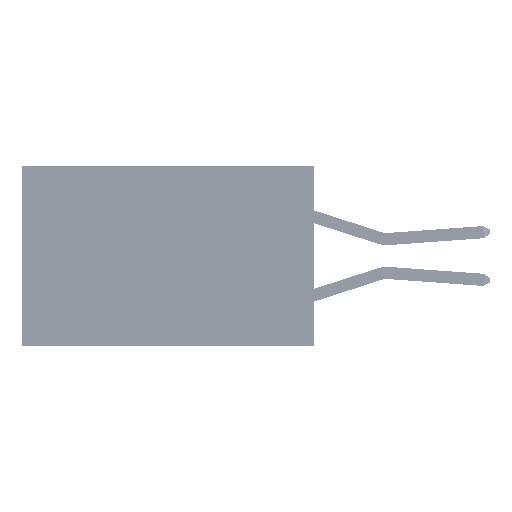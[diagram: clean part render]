
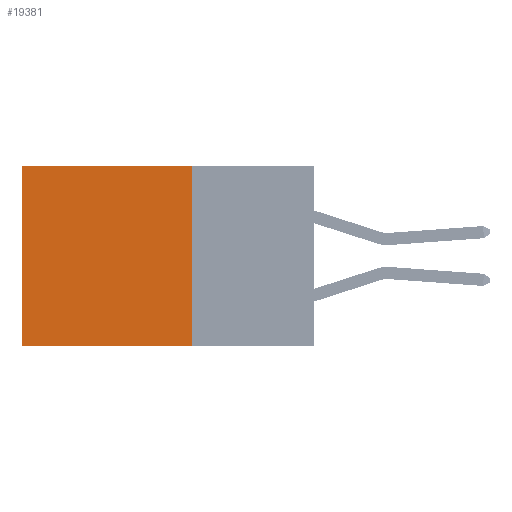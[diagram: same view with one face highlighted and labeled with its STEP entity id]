
A CAD part, left-side view. The second image highlights one B-rep face of the part: STEP entity #19381.
In plain terms, the highlighted planar face has unit normal (-1, 0, 0).
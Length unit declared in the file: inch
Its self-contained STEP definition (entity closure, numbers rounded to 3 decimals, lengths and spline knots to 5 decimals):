
#214 = VERTEX_POINT ( 'NONE', #16503 ) ;
#2511 = ORIENTED_EDGE ( 'NONE', *, *, #20797, .T. ) ;
#3093 = PLANE ( 'NONE',  #17637 ) ;
#3912 = DIRECTION ( 'NONE',  ( 0., 0., -1. ) ) ;
#6927 = DIRECTION ( 'NONE',  ( 1., 0., 0. ) ) ;
#7312 = DIRECTION ( 'NONE',  ( 0., 1., 0. ) ) ;
#7594 = LINE ( 'NONE', #33003, #8791 ) ;
#8791 = VECTOR ( 'NONE', #10518, 39.37008 ) ;
#9837 = LINE ( 'NONE', #20962, #28636 ) ;
#10518 = DIRECTION ( 'NONE',  ( 0., 0., -1. ) ) ;
#10576 = CARTESIAN_POINT ( 'NONE',  ( 0.2875, 0.25, 0. ) ) ;
#12456 = VERTEX_POINT ( 'NONE', #47405 ) ;
#16503 = CARTESIAN_POINT ( 'NONE',  ( 0.2875, 0.6, 0. ) ) ;
#17637 = AXIS2_PLACEMENT_3D ( 'NONE', #10576, #6927, #33221 ) ;
#19381 = ADVANCED_FACE ( 'NONE', ( #26759 ), #3093, .F. ) ;
#19738 = VERTEX_POINT ( 'NONE', #38756 ) ;
#20797 = EDGE_CURVE ( 'NONE', #19738, #214, #40664, .T. ) ;
#20962 = CARTESIAN_POINT ( 'NONE',  ( 0.2875, 0.25, -0.37 ) ) ;
#21660 = VERTEX_POINT ( 'NONE', #47685 ) ;
#22228 = ORIENTED_EDGE ( 'NONE', *, *, #28648, .F. ) ;
#26374 = VECTOR ( 'NONE', #3912, 39.37008 ) ;
#26486 = CARTESIAN_POINT ( 'NONE',  ( 0.2875, 0.6, 0. ) ) ;
#26759 = FACE_OUTER_BOUND ( 'NONE', #41719, .T. ) ;
#28636 = VECTOR ( 'NONE', #35816, 39.37008 ) ;
#28648 = EDGE_CURVE ( 'NONE', #12456, #21660, #9837, .T. ) ;
#30365 = ORIENTED_EDGE ( 'NONE', *, *, #33976, .T. ) ;
#30696 = VECTOR ( 'NONE', #7312, 39.37008 ) ;
#33003 = CARTESIAN_POINT ( 'NONE',  ( 0.2875, 0.25, 0. ) ) ;
#33221 = DIRECTION ( 'NONE',  ( 0., 0., -1. ) ) ;
#33976 = EDGE_CURVE ( 'NONE', #214, #21660, #35166, .T. ) ;
#35166 = LINE ( 'NONE', #26486, #26374 ) ;
#35816 = DIRECTION ( 'NONE',  ( 0., 1., 0. ) ) ;
#38756 = CARTESIAN_POINT ( 'NONE',  ( 0.2875, 0.25, 0. ) ) ;
#40664 = LINE ( 'NONE', #44677, #30696 ) ;
#41029 = EDGE_CURVE ( 'NONE', #19738, #12456, #7594, .T. ) ;
#41719 = EDGE_LOOP ( 'NONE', ( #30365, #22228, #47009, #2511 ) ) ;
#44677 = CARTESIAN_POINT ( 'NONE',  ( 0.2875, 0.25, 0. ) ) ;
#47009 = ORIENTED_EDGE ( 'NONE', *, *, #41029, .F. ) ;
#47405 = CARTESIAN_POINT ( 'NONE',  ( 0.2875, 0.25, -0.37 ) ) ;
#47685 = CARTESIAN_POINT ( 'NONE',  ( 0.2875, 0.6, -0.37 ) ) ;
